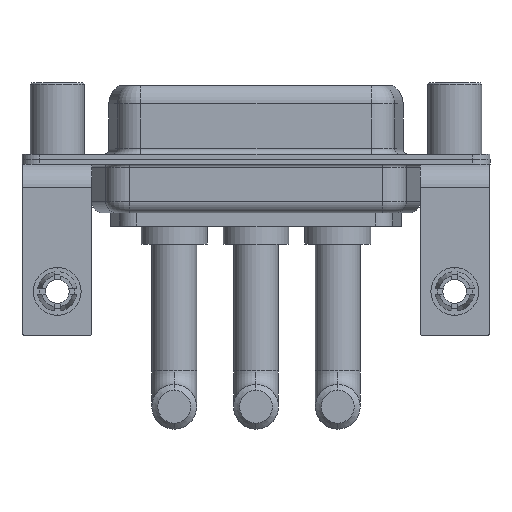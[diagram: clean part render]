
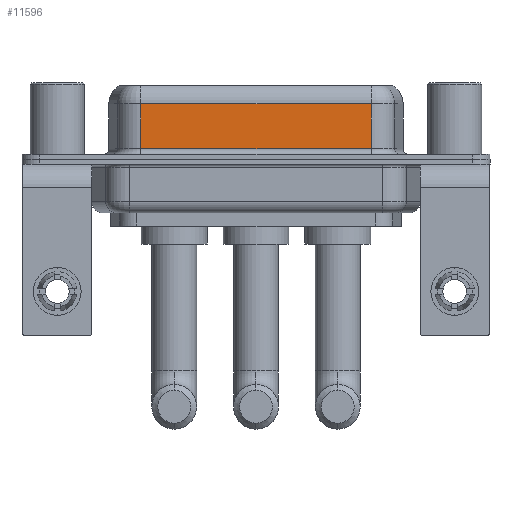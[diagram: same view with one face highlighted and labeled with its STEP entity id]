
A CAD part, front view. The second image highlights one B-rep face of the part: STEP entity #11596.
In plain terms, the highlighted planar face has unit normal (0, -1, 0).
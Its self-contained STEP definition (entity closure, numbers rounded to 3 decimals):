
#24 = LINE ( 'NONE', #14498, #10787 ) ;
#172 = VECTOR ( 'NONE', #10946, 1000. ) ;
#320 = EDGE_CURVE ( 'NONE', #15741, #1213, #6035, .T. ) ;
#763 = ORIENTED_EDGE ( 'NONE', *, *, #320, .T. ) ;
#918 = EDGE_LOOP ( 'NONE', ( #7425, #763, #5391, #12051 ) ) ;
#1126 = CARTESIAN_POINT ( 'NONE',  ( 7.013, -3.95, 6.4 ) ) ;
#1213 = VERTEX_POINT ( 'NONE', #4308 ) ;
#1804 = CARTESIAN_POINT ( 'NONE',  ( 7.013, -3.95, 0.9 ) ) ;
#3237 = CARTESIAN_POINT ( 'NONE',  ( 26.287, -3.95, 4.65 ) ) ;
#4308 = CARTESIAN_POINT ( 'NONE',  ( 7.013, -3.95, 4.65 ) ) ;
#4608 = DIRECTION ( 'NONE',  ( 0., 1., 0. ) ) ;
#4899 = DIRECTION ( 'NONE',  ( 1., 0., 0. ) ) ;
#5391 = ORIENTED_EDGE ( 'NONE', *, *, #14426, .T. ) ;
#5490 = AXIS2_PLACEMENT_3D ( 'NONE', #15655, #4608, #9530 ) ;
#5603 = EDGE_CURVE ( 'NONE', #11120, #15181, #24, .T. ) ;
#5820 = PLANE ( 'NONE',  #5490 ) ;
#6035 = LINE ( 'NONE', #9740, #172 ) ;
#6088 = LINE ( 'NONE', #15757, #15071 ) ;
#6090 = LINE ( 'NONE', #1126, #15869 ) ;
#7425 = ORIENTED_EDGE ( 'NONE', *, *, #13112, .F. ) ;
#9108 = CARTESIAN_POINT ( 'NONE',  ( 26.287, -3.95, 0.9 ) ) ;
#9530 = DIRECTION ( 'NONE',  ( 0., 0., 1. ) ) ;
#9740 = CARTESIAN_POINT ( 'NONE',  ( 26.287, -3.95, 4.65 ) ) ;
#10787 = VECTOR ( 'NONE', #4899, 1000. ) ;
#10946 = DIRECTION ( 'NONE',  ( -1., 0., 0. ) ) ;
#11120 = VERTEX_POINT ( 'NONE', #1804 ) ;
#11596 = ADVANCED_FACE ( 'NONE', ( #15497 ), #5820, .F. ) ;
#12051 = ORIENTED_EDGE ( 'NONE', *, *, #5603, .T. ) ;
#12131 = DIRECTION ( 'NONE',  ( 0., 0., -1. ) ) ;
#13112 = EDGE_CURVE ( 'NONE', #15741, #15181, #6088, .T. ) ;
#14426 = EDGE_CURVE ( 'NONE', #1213, #11120, #6090, .T. ) ;
#14498 = CARTESIAN_POINT ( 'NONE',  ( 26.287, -3.95, 0.9 ) ) ;
#15071 = VECTOR ( 'NONE', #12131, 1000. ) ;
#15181 = VERTEX_POINT ( 'NONE', #9108 ) ;
#15497 = FACE_OUTER_BOUND ( 'NONE', #918, .T. ) ;
#15655 = CARTESIAN_POINT ( 'NONE',  ( 26.287, -3.95, 6.4 ) ) ;
#15741 = VERTEX_POINT ( 'NONE', #3237 ) ;
#15757 = CARTESIAN_POINT ( 'NONE',  ( 26.287, -3.95, 6.4 ) ) ;
#15869 = VECTOR ( 'NONE', #15908, 1000. ) ;
#15908 = DIRECTION ( 'NONE',  ( 0., 0., -1. ) ) ;
